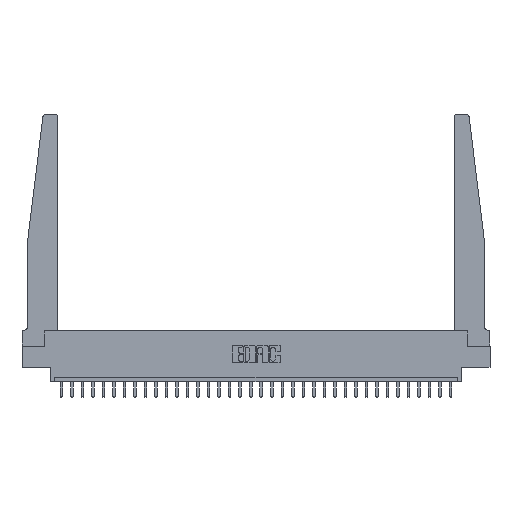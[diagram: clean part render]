
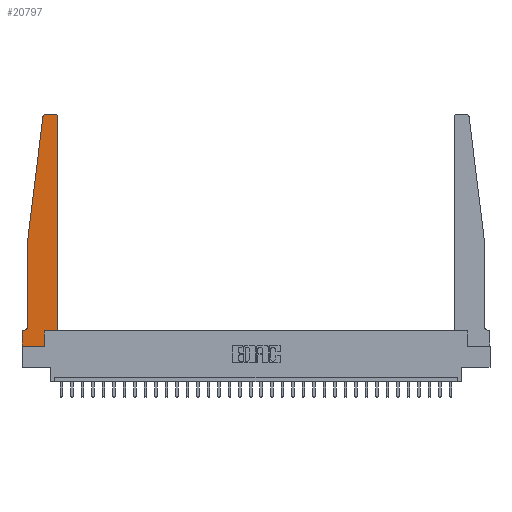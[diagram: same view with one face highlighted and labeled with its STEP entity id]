
A CAD part, top view. The second image highlights one B-rep face of the part: STEP entity #20797.
In plain terms, the highlighted planar face has unit normal (0, 0, 1).
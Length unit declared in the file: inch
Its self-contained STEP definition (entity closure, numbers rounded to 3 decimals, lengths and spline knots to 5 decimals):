
#1 = LINE ( 'NONE', #11697, #25265 ) ;
#91 = LINE ( 'NONE', #14035, #13908 ) ;
#308 = CARTESIAN_POINT ( 'NONE',  ( 0.425, 0.18, 0.37 ) ) ;
#325 = CARTESIAN_POINT ( 'NONE',  ( 0.065, 1.25, 0.37 ) ) ;
#423 = DIRECTION ( 'NONE',  ( -1., 0., 0. ) ) ;
#537 = CARTESIAN_POINT ( 'NONE',  ( 0., 0., 0.37 ) ) ;
#1173 = EDGE_CURVE ( 'NONE', #14220, #9912, #8456, .T. ) ;
#2003 = VECTOR ( 'NONE', #9336, 39.37008 ) ;
#2204 = EDGE_CURVE ( 'NONE', #20309, #29196, #5803, .T. ) ;
#2325 = EDGE_CURVE ( 'NONE', #6606, #14844, #27466, .T. ) ;
#2401 = PLANE ( 'NONE',  #16783 ) ;
#2661 = EDGE_LOOP ( 'NONE', ( #14055, #10974, #25269, #9137, #9005, #23556, #5946, #7260, #24639, #24148, #17870, #25613 ) ) ;
#2752 = AXIS2_PLACEMENT_3D ( 'NONE', #4149, #15549, #24536 ) ;
#3304 = EDGE_CURVE ( 'NONE', #9912, #25681, #16074, .T. ) ;
#3708 = DIRECTION ( 'NONE',  ( 0., 1., 0. ) ) ;
#4149 = CARTESIAN_POINT ( 'NONE',  ( 0.27653, 2.72, 0.37 ) ) ;
#4565 = CARTESIAN_POINT ( 'NONE',  ( 0.2605, 0.18, 0.37 ) ) ;
#4660 = DIRECTION ( 'NONE',  ( 0., 0., 1. ) ) ;
#4737 = CARTESIAN_POINT ( 'NONE',  ( 0.065, 0.2375, 0.37 ) ) ;
#5803 = LINE ( 'NONE', #12569, #29155 ) ;
#5946 = ORIENTED_EDGE ( 'NONE', *, *, #17265, .T. ) ;
#5976 = CARTESIAN_POINT ( 'NONE',  ( 0.395, 2.72, 0.37 ) ) ;
#6606 = VERTEX_POINT ( 'NONE', #19066 ) ;
#7260 = ORIENTED_EDGE ( 'NONE', *, *, #21232, .T. ) ;
#8301 = CARTESIAN_POINT ( 'NONE',  ( 0.065, 1.25, 0.37 ) ) ;
#8456 = LINE ( 'NONE', #8301, #11312 ) ;
#8509 = CARTESIAN_POINT ( 'NONE',  ( 0.2605, 0., 0.37 ) ) ;
#8614 = DIRECTION ( 'NONE',  ( -0.122, -0.992, 0. ) ) ;
#8999 = VECTOR ( 'NONE', #25638, 39.37008 ) ;
#9005 = ORIENTED_EDGE ( 'NONE', *, *, #26432, .T. ) ;
#9131 = CARTESIAN_POINT ( 'NONE',  ( 0.065, 1.25, 0.37 ) ) ;
#9137 = ORIENTED_EDGE ( 'NONE', *, *, #3304, .T. ) ;
#9336 = DIRECTION ( 'NONE',  ( 0., -1., 0. ) ) ;
#9912 = VERTEX_POINT ( 'NONE', #9131 ) ;
#10032 = CARTESIAN_POINT ( 'NONE',  ( 0., 0.1875, 0.37 ) ) ;
#10974 = ORIENTED_EDGE ( 'NONE', *, *, #28915, .T. ) ;
#11312 = VECTOR ( 'NONE', #8614, 39.37008 ) ;
#11697 = CARTESIAN_POINT ( 'NONE',  ( 0.25, 2.75, 0.37 ) ) ;
#11920 = CIRCLE ( 'NONE', #28599, 0.05 ) ;
#11992 = EDGE_CURVE ( 'NONE', #27350, #20309, #26321, .T. ) ;
#12569 = CARTESIAN_POINT ( 'NONE',  ( 0.425, 0.18, 0.37 ) ) ;
#13357 = FACE_OUTER_BOUND ( 'NONE', #2661, .T. ) ;
#13908 = VECTOR ( 'NONE', #18683, 39.37008 ) ;
#14035 = CARTESIAN_POINT ( 'NONE',  ( 0., 0., 0.37 ) ) ;
#14055 = ORIENTED_EDGE ( 'NONE', *, *, #26987, .T. ) ;
#14173 = CARTESIAN_POINT ( 'NONE',  ( 0.395, 2.75, 0.37 ) ) ;
#14220 = VERTEX_POINT ( 'NONE', #27428 ) ;
#14844 = VERTEX_POINT ( 'NONE', #10032 ) ;
#15040 = VERTEX_POINT ( 'NONE', #537 ) ;
#15448 = CARTESIAN_POINT ( 'NONE',  ( 0.015, 0.2375, 0.37 ) ) ;
#15549 = DIRECTION ( 'NONE',  ( 0., 0., 1. ) ) ;
#15893 = DIRECTION ( 'NONE',  ( 1., 0., 0. ) ) ;
#16074 = LINE ( 'NONE', #325, #2003 ) ;
#16642 = DIRECTION ( 'NONE',  ( 0., 1., 0. ) ) ;
#16783 = AXIS2_PLACEMENT_3D ( 'NONE', #20691, #4660, #15893 ) ;
#16972 = LINE ( 'NONE', #27711, #8999 ) ;
#17180 = DIRECTION ( 'NONE',  ( 1., 0., 0. ) ) ;
#17255 = VECTOR ( 'NONE', #21218, 39.37008 ) ;
#17265 = EDGE_CURVE ( 'NONE', #14844, #15040, #16972, .T. ) ;
#17353 = DIRECTION ( 'NONE',  ( 1., 0., 0. ) ) ;
#17870 = ORIENTED_EDGE ( 'NONE', *, *, #26141, .T. ) ;
#18683 = DIRECTION ( 'NONE',  ( 1., 0., 0. ) ) ;
#19066 = CARTESIAN_POINT ( 'NONE',  ( 0.015, 0.1875, 0.37 ) ) ;
#20063 = VERTEX_POINT ( 'NONE', #14173 ) ;
#20309 = VERTEX_POINT ( 'NONE', #4565 ) ;
#20514 = DIRECTION ( 'NONE',  ( -1., 0., 0. ) ) ;
#20662 = CIRCLE ( 'NONE', #24504, 0.03 ) ;
#20691 = CARTESIAN_POINT ( 'NONE',  ( 0., 0.1875, 0.37 ) ) ;
#20797 = ADVANCED_FACE ( 'NONE', ( #13357 ), #2401, .T. ) ;
#20947 = CIRCLE ( 'NONE', #2752, 0.03 ) ;
#21218 = DIRECTION ( 'NONE',  ( -1., 0., 0. ) ) ;
#21232 = EDGE_CURVE ( 'NONE', #15040, #27350, #91, .T. ) ;
#21513 = VECTOR ( 'NONE', #16642, 39.37008 ) ;
#22754 = EDGE_CURVE ( 'NONE', #24055, #20063, #20662, .T. ) ;
#23556 = ORIENTED_EDGE ( 'NONE', *, *, #2325, .T. ) ;
#24055 = VERTEX_POINT ( 'NONE', #24425 ) ;
#24148 = ORIENTED_EDGE ( 'NONE', *, *, #2204, .T. ) ;
#24248 = CARTESIAN_POINT ( 'NONE',  ( 0.2605, 0.18, 0.37 ) ) ;
#24392 = DIRECTION ( 'NONE',  ( 0., 0., 1. ) ) ;
#24425 = CARTESIAN_POINT ( 'NONE',  ( 0.425, 2.72, 0.37 ) ) ;
#24504 = AXIS2_PLACEMENT_3D ( 'NONE', #5976, #24392, #17353 ) ;
#24536 = DIRECTION ( 'NONE',  ( 1., 0., 0. ) ) ;
#24639 = ORIENTED_EDGE ( 'NONE', *, *, #11992, .T. ) ;
#25265 = VECTOR ( 'NONE', #423, 39.37008 ) ;
#25269 = ORIENTED_EDGE ( 'NONE', *, *, #1173, .T. ) ;
#25613 = ORIENTED_EDGE ( 'NONE', *, *, #22754, .T. ) ;
#25638 = DIRECTION ( 'NONE',  ( 0., -1., 0. ) ) ;
#25681 = VERTEX_POINT ( 'NONE', #4737 ) ;
#25826 = CARTESIAN_POINT ( 'NONE',  ( 0.065, 0.1875, 0.37 ) ) ;
#26141 = EDGE_CURVE ( 'NONE', #29196, #24055, #27987, .T. ) ;
#26321 = LINE ( 'NONE', #24248, #28374 ) ;
#26432 = EDGE_CURVE ( 'NONE', #25681, #6606, #11920, .T. ) ;
#26987 = EDGE_CURVE ( 'NONE', #20063, #27900, #1, .T. ) ;
#27350 = VERTEX_POINT ( 'NONE', #8509 ) ;
#27428 = CARTESIAN_POINT ( 'NONE',  ( 0.24675, 2.72367, 0.37 ) ) ;
#27466 = LINE ( 'NONE', #25826, #17255 ) ;
#27711 = CARTESIAN_POINT ( 'NONE',  ( 0., 0., 0.37 ) ) ;
#27900 = VERTEX_POINT ( 'NONE', #28339 ) ;
#27987 = LINE ( 'NONE', #308, #21513 ) ;
#28339 = CARTESIAN_POINT ( 'NONE',  ( 0.27653, 2.75, 0.37 ) ) ;
#28374 = VECTOR ( 'NONE', #3708, 39.37008 ) ;
#28599 = AXIS2_PLACEMENT_3D ( 'NONE', #15448, #29337, #20514 ) ;
#28915 = EDGE_CURVE ( 'NONE', #27900, #14220, #20947, .T. ) ;
#29155 = VECTOR ( 'NONE', #17180, 39.37008 ) ;
#29196 = VERTEX_POINT ( 'NONE', #29563 ) ;
#29337 = DIRECTION ( 'NONE',  ( 0., 0., -1. ) ) ;
#29563 = CARTESIAN_POINT ( 'NONE',  ( 0.425, 0.18, 0.37 ) ) ;
